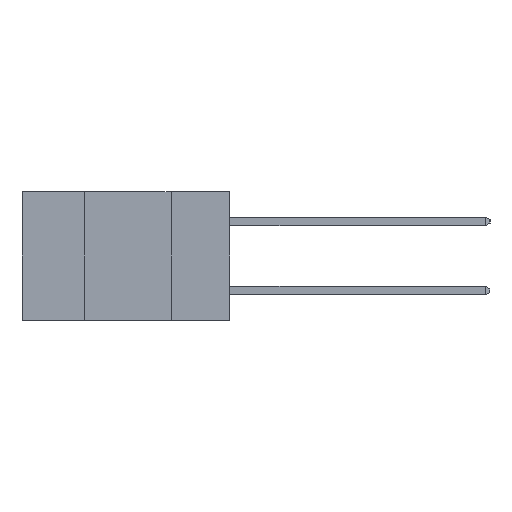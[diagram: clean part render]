
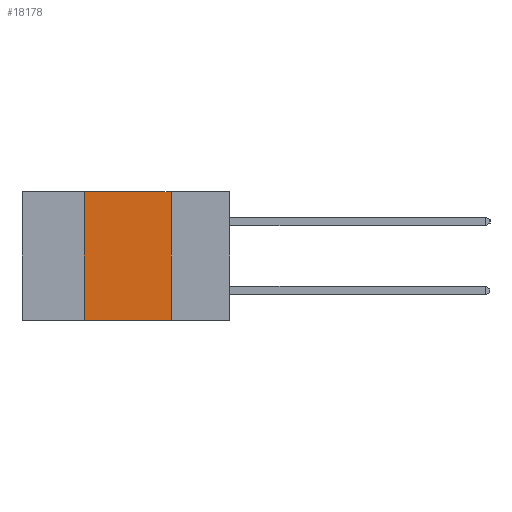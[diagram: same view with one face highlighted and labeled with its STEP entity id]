
A CAD part, left-side view. The second image highlights one B-rep face of the part: STEP entity #18178.
In plain terms, the highlighted planar face has unit normal (-1, 0, 0).
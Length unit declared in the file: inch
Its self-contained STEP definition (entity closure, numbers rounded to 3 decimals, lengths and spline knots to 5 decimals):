
#556 = DIRECTION ( 'NONE',  ( 0., -1., 0. ) ) ;
#733 = VECTOR ( 'NONE', #12000, 39.37008 ) ;
#915 = VERTEX_POINT ( 'NONE', #18453 ) ;
#1030 = LINE ( 'NONE', #16151, #20654 ) ;
#1929 = DIRECTION ( 'NONE',  ( 1., 0., 0. ) ) ;
#1960 = VECTOR ( 'NONE', #19702, 39.37008 ) ;
#2160 = VERTEX_POINT ( 'NONE', #20380 ) ;
#3800 = PLANE ( 'NONE',  #15976 ) ;
#4071 = VERTEX_POINT ( 'NONE', #4865 ) ;
#4178 = CARTESIAN_POINT ( 'NONE',  ( 0., 0.42, 0. ) ) ;
#4414 = LINE ( 'NONE', #17733, #1960 ) ;
#4865 = CARTESIAN_POINT ( 'NONE',  ( 0., 0.42, -0.37 ) ) ;
#5938 = LINE ( 'NONE', #4178, #733 ) ;
#7131 = VECTOR ( 'NONE', #17190, 39.37008 ) ;
#7752 = LINE ( 'NONE', #9368, #7131 ) ;
#7974 = ORIENTED_EDGE ( 'NONE', *, *, #25319, .T. ) ;
#9368 = CARTESIAN_POINT ( 'NONE',  ( 0., 0.17, 0. ) ) ;
#9626 = EDGE_CURVE ( 'NONE', #915, #2160, #1030, .T. ) ;
#11227 = ORIENTED_EDGE ( 'NONE', *, *, #25399, .F. ) ;
#12000 = DIRECTION ( 'NONE',  ( 0., 0., 1. ) ) ;
#13307 = VERTEX_POINT ( 'NONE', #19429 ) ;
#14139 = ORIENTED_EDGE ( 'NONE', *, *, #15849, .F. ) ;
#15311 = CARTESIAN_POINT ( 'NONE',  ( 0., 0.6, 0. ) ) ;
#15632 = DIRECTION ( 'NONE',  ( 0., 0., -1. ) ) ;
#15849 = EDGE_CURVE ( 'NONE', #2160, #13307, #7752, .T. ) ;
#15976 = AXIS2_PLACEMENT_3D ( 'NONE', #15311, #1929, #15632 ) ;
#16151 = CARTESIAN_POINT ( 'NONE',  ( 0., 0.6, 0. ) ) ;
#16517 = EDGE_LOOP ( 'NONE', ( #14139, #22576, #11227, #7974 ) ) ;
#17190 = DIRECTION ( 'NONE',  ( 0., 0., -1. ) ) ;
#17733 = CARTESIAN_POINT ( 'NONE',  ( 0., 0.6, -0.37 ) ) ;
#18178 = ADVANCED_FACE ( 'NONE', ( #19600 ), #3800, .F. ) ;
#18453 = CARTESIAN_POINT ( 'NONE',  ( 0., 0.42, 0. ) ) ;
#19429 = CARTESIAN_POINT ( 'NONE',  ( 0., 0.17, -0.37 ) ) ;
#19600 = FACE_OUTER_BOUND ( 'NONE', #16517, .T. ) ;
#19702 = DIRECTION ( 'NONE',  ( 0., -1., 0. ) ) ;
#20380 = CARTESIAN_POINT ( 'NONE',  ( 0., 0.17, 0. ) ) ;
#20654 = VECTOR ( 'NONE', #556, 39.37008 ) ;
#22576 = ORIENTED_EDGE ( 'NONE', *, *, #9626, .F. ) ;
#25319 = EDGE_CURVE ( 'NONE', #4071, #13307, #4414, .T. ) ;
#25399 = EDGE_CURVE ( 'NONE', #4071, #915, #5938, .T. ) ;
